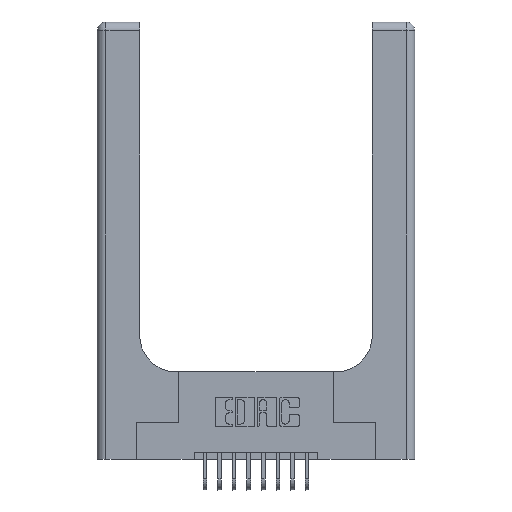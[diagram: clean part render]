
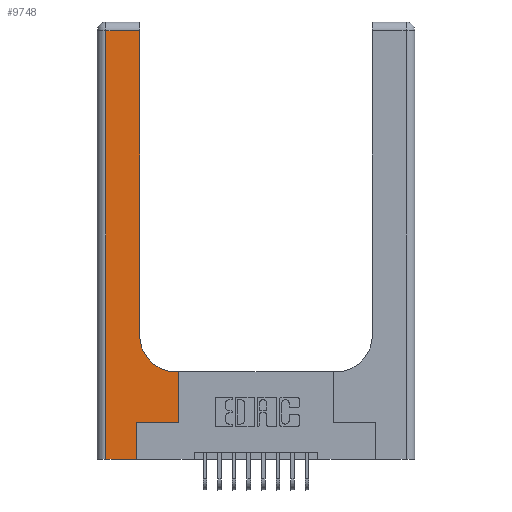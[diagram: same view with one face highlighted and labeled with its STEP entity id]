
A CAD part, top view. The second image highlights one B-rep face of the part: STEP entity #9748.
In plain terms, the highlighted planar face has unit normal (0, 0, 1).
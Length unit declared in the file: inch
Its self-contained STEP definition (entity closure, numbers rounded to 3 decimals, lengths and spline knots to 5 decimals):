
#237 = ORIENTED_EDGE ( 'NONE', *, *, #14079, .T. ) ;
#339 = ORIENTED_EDGE ( 'NONE', *, *, #8744, .T. ) ;
#849 = CARTESIAN_POINT ( 'NONE',  ( 0.5585, 0.6, 0.37 ) ) ;
#917 = EDGE_CURVE ( 'NONE', #13388, #13480, #5703, .T. ) ;
#1068 = VERTEX_POINT ( 'NONE', #8727 ) ;
#1170 = LINE ( 'NONE', #15861, #5265 ) ;
#1325 = DIRECTION ( 'NONE',  ( 0., 0., -1. ) ) ;
#1389 = EDGE_CURVE ( 'NONE', #3999, #1068, #14233, .T. ) ;
#1591 = CARTESIAN_POINT ( 'NONE',  ( 0.269, 0.25, 0.37 ) ) ;
#2042 = DIRECTION ( 'NONE',  ( 0., -1., 0. ) ) ;
#2048 = PLANE ( 'NONE',  #5469 ) ;
#2771 = VECTOR ( 'NONE', #7697, 39.37008 ) ;
#3109 = VECTOR ( 'NONE', #7169, 39.37008 ) ;
#3268 = VECTOR ( 'NONE', #6197, 39.37008 ) ;
#3999 = VERTEX_POINT ( 'NONE', #4648 ) ;
#4218 = VECTOR ( 'NONE', #15235, 39.37008 ) ;
#4222 = DIRECTION ( 'NONE',  ( 0., 1., 0. ) ) ;
#4318 = CARTESIAN_POINT ( 'NONE',  ( 0.2915, 3., 0.37 ) ) ;
#4340 = CARTESIAN_POINT ( 'NONE',  ( 0.2915, 2.94, 0.37 ) ) ;
#4648 = CARTESIAN_POINT ( 'NONE',  ( 0.06, 2.94, 0.37 ) ) ;
#4691 = AXIS2_PLACEMENT_3D ( 'NONE', #10937, #1325, #5531 ) ;
#4694 = DIRECTION ( 'NONE',  ( 0., 0., -1. ) ) ;
#5265 = VECTOR ( 'NONE', #11849, 39.37008 ) ;
#5469 = AXIS2_PLACEMENT_3D ( 'NONE', #12982, #4694, #7432 ) ;
#5531 = DIRECTION ( 'NONE',  ( 1., 0., 0. ) ) ;
#5703 = LINE ( 'NONE', #11287, #3109 ) ;
#5980 = ORIENTED_EDGE ( 'NONE', *, *, #9819, .T. ) ;
#6056 = EDGE_CURVE ( 'NONE', #11758, #11863, #7320, .T. ) ;
#6167 = VERTEX_POINT ( 'NONE', #8546 ) ;
#6197 = DIRECTION ( 'NONE',  ( -1., 0., 0. ) ) ;
#6357 = DIRECTION ( 'NONE',  ( 1., 0., 0. ) ) ;
#6959 = LINE ( 'NONE', #4318, #4218 ) ;
#7165 = VERTEX_POINT ( 'NONE', #4340 ) ;
#7169 = DIRECTION ( 'NONE',  ( 1., 0., 0. ) ) ;
#7278 = LINE ( 'NONE', #10382, #14550 ) ;
#7310 = CARTESIAN_POINT ( 'NONE',  ( 0.06, 3., 0.37 ) ) ;
#7320 = LINE ( 'NONE', #11746, #3268 ) ;
#7432 = DIRECTION ( 'NONE',  ( -1., 0., 0. ) ) ;
#7692 = LINE ( 'NONE', #10298, #2771 ) ;
#7697 = DIRECTION ( 'NONE',  ( 0., 1., 0. ) ) ;
#8546 = CARTESIAN_POINT ( 'NONE',  ( 0.269, 0., 0.37 ) ) ;
#8727 = CARTESIAN_POINT ( 'NONE',  ( 0.06, 0., 0.37 ) ) ;
#8744 = EDGE_CURVE ( 'NONE', #10016, #7165, #6959, .T. ) ;
#9748 = ADVANCED_FACE ( 'NONE', ( #12282 ), #2048, .F. ) ;
#9809 = CARTESIAN_POINT ( 'NONE',  ( 0.5585, 0.25, 0.37 ) ) ;
#9819 = EDGE_CURVE ( 'NONE', #7165, #3999, #1170, .T. ) ;
#9964 = EDGE_LOOP ( 'NONE', ( #339, #5980, #17640, #11075, #14460, #14385, #11170, #11457, #237 ) ) ;
#10016 = VERTEX_POINT ( 'NONE', #13848 ) ;
#10298 = CARTESIAN_POINT ( 'NONE',  ( 0.5585, 0.25, 0.37 ) ) ;
#10382 = CARTESIAN_POINT ( 'NONE',  ( 0., 0., 0.37 ) ) ;
#10870 = CARTESIAN_POINT ( 'NONE',  ( 0.269, 0., 0.37 ) ) ;
#10937 = CARTESIAN_POINT ( 'NONE',  ( 0.5415, 0.85, 0.37 ) ) ;
#11075 = ORIENTED_EDGE ( 'NONE', *, *, #12957, .T. ) ;
#11170 = ORIENTED_EDGE ( 'NONE', *, *, #13422, .T. ) ;
#11287 = CARTESIAN_POINT ( 'NONE',  ( 0.269, 0.25, 0.37 ) ) ;
#11457 = ORIENTED_EDGE ( 'NONE', *, *, #6056, .T. ) ;
#11746 = CARTESIAN_POINT ( 'NONE',  ( 0.2915, 0.6, 0.37 ) ) ;
#11758 = VERTEX_POINT ( 'NONE', #849 ) ;
#11849 = DIRECTION ( 'NONE',  ( -1., 0., 0. ) ) ;
#11863 = VERTEX_POINT ( 'NONE', #11974 ) ;
#11974 = CARTESIAN_POINT ( 'NONE',  ( 0.5415, 0.6, 0.37 ) ) ;
#12282 = FACE_OUTER_BOUND ( 'NONE', #9964, .T. ) ;
#12957 = EDGE_CURVE ( 'NONE', #1068, #6167, #7278, .T. ) ;
#12982 = CARTESIAN_POINT ( 'NONE',  ( 0., 3., 0.37 ) ) ;
#13388 = VERTEX_POINT ( 'NONE', #1591 ) ;
#13422 = EDGE_CURVE ( 'NONE', #13480, #11758, #7692, .T. ) ;
#13480 = VERTEX_POINT ( 'NONE', #9809 ) ;
#13848 = CARTESIAN_POINT ( 'NONE',  ( 0.2915, 0.85, 0.37 ) ) ;
#14079 = EDGE_CURVE ( 'NONE', #11863, #10016, #17073, .T. ) ;
#14233 = LINE ( 'NONE', #7310, #15966 ) ;
#14385 = ORIENTED_EDGE ( 'NONE', *, *, #917, .T. ) ;
#14460 = ORIENTED_EDGE ( 'NONE', *, *, #17029, .T. ) ;
#14550 = VECTOR ( 'NONE', #6357, 39.37008 ) ;
#15235 = DIRECTION ( 'NONE',  ( 0., 1., 0. ) ) ;
#15755 = LINE ( 'NONE', #10870, #16609 ) ;
#15861 = CARTESIAN_POINT ( 'NONE',  ( 0., 2.94, 0.37 ) ) ;
#15966 = VECTOR ( 'NONE', #2042, 39.37008 ) ;
#16609 = VECTOR ( 'NONE', #4222, 39.37008 ) ;
#17029 = EDGE_CURVE ( 'NONE', #6167, #13388, #15755, .T. ) ;
#17073 = CIRCLE ( 'NONE', #4691, 0.25 ) ;
#17640 = ORIENTED_EDGE ( 'NONE', *, *, #1389, .T. ) ;
